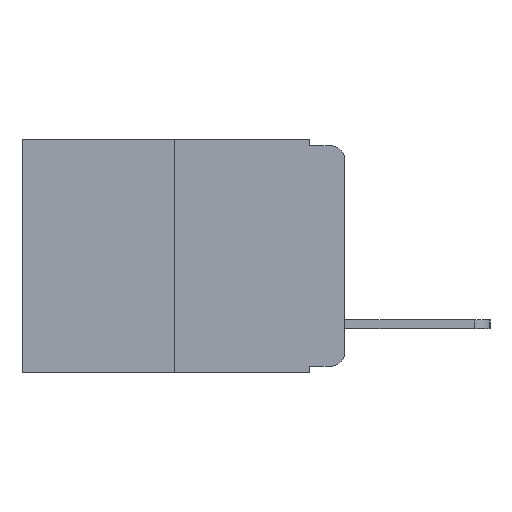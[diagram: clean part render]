
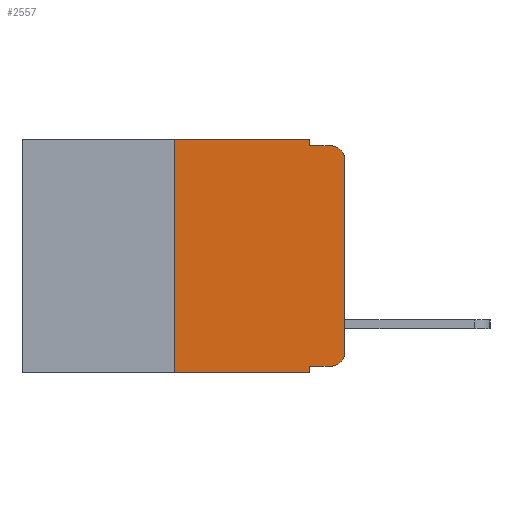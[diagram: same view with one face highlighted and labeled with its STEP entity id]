
A CAD part, left-side view. The second image highlights one B-rep face of the part: STEP entity #2557.
In plain terms, the highlighted planar face has unit normal (-1, 0, 0).
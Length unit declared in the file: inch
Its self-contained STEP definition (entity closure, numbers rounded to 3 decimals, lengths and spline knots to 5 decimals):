
#307 = DIRECTION ( 'NONE',  ( 0., -1., 0. ) ) ;
#320 = EDGE_CURVE ( 'NONE', #17884, #18486, #10785, .T. ) ;
#479 = VERTEX_POINT ( 'NONE', #16959 ) ;
#523 = CARTESIAN_POINT ( 'NONE',  ( 0., 0.051, 0. ) ) ;
#630 = LINE ( 'NONE', #13786, #11543 ) ;
#635 = VECTOR ( 'NONE', #307, 39.37008 ) ;
#1084 = ORIENTED_EDGE ( 'NONE', *, *, #12898, .T. ) ;
#1137 = CARTESIAN_POINT ( 'NONE',  ( 0., 0.473, 0. ) ) ;
#1275 = CIRCLE ( 'NONE', #4536, 0.02 ) ;
#1301 = VERTEX_POINT ( 'NONE', #3215 ) ;
#1553 = DIRECTION ( 'NONE',  ( -1., 0., 0. ) ) ;
#1651 = CARTESIAN_POINT ( 'NONE',  ( 0., 0.051, -0.01 ) ) ;
#2557 = ADVANCED_FACE ( 'NONE', ( #8047 ), #15095, .F. ) ;
#2759 = CARTESIAN_POINT ( 'NONE',  ( 0., 0.051, -0.01 ) ) ;
#2769 = DIRECTION ( 'NONE',  ( 0., 0., 1. ) ) ;
#2838 = VERTEX_POINT ( 'NONE', #18461 ) ;
#2897 = DIRECTION ( 'NONE',  ( 0., -1., 0. ) ) ;
#2990 = DIRECTION ( 'NONE',  ( 0., -1., 0. ) ) ;
#3191 = ORIENTED_EDGE ( 'NONE', *, *, #7468, .F. ) ;
#3215 = CARTESIAN_POINT ( 'NONE',  ( 0., 0.25, 0. ) ) ;
#3253 = ORIENTED_EDGE ( 'NONE', *, *, #10333, .F. ) ;
#3275 = VECTOR ( 'NONE', #9499, 39.37008 ) ;
#3649 = EDGE_CURVE ( 'NONE', #1301, #15613, #4706, .T. ) ;
#4244 = VECTOR ( 'NONE', #2990, 39.37008 ) ;
#4536 = AXIS2_PLACEMENT_3D ( 'NONE', #10446, #1553, #11887 ) ;
#4706 = LINE ( 'NONE', #1137, #4244 ) ;
#5026 = VECTOR ( 'NONE', #17698, 39.37008 ) ;
#5345 = LINE ( 'NONE', #15809, #12645 ) ;
#5619 = CARTESIAN_POINT ( 'NONE',  ( 0., 0.051, 0. ) ) ;
#5855 = CARTESIAN_POINT ( 'NONE',  ( 0., 0.02, -0.03 ) ) ;
#6069 = ORIENTED_EDGE ( 'NONE', *, *, #12273, .T. ) ;
#6139 = CARTESIAN_POINT ( 'NONE',  ( 0., 0.02, -0.333 ) ) ;
#6470 = EDGE_CURVE ( 'NONE', #17884, #9481, #6819, .T. ) ;
#6799 = ORIENTED_EDGE ( 'NONE', *, *, #6470, .F. ) ;
#6819 = LINE ( 'NONE', #523, #3275 ) ;
#7158 = CARTESIAN_POINT ( 'NONE',  ( 0., 0.25, -0.343 ) ) ;
#7377 = DIRECTION ( 'NONE',  ( 0., 0., -1. ) ) ;
#7468 = EDGE_CURVE ( 'NONE', #13738, #1301, #5345, .T. ) ;
#8047 = FACE_OUTER_BOUND ( 'NONE', #12442, .T. ) ;
#8198 = LINE ( 'NONE', #9336, #635 ) ;
#8646 = CARTESIAN_POINT ( 'NONE',  ( 0., 0., -0.313 ) ) ;
#9336 = CARTESIAN_POINT ( 'NONE',  ( 0., 0.473, -0.343 ) ) ;
#9407 = EDGE_CURVE ( 'NONE', #15613, #11278, #12786, .T. ) ;
#9481 = VERTEX_POINT ( 'NONE', #10815 ) ;
#9499 = DIRECTION ( 'NONE',  ( 0., 0., -1. ) ) ;
#9705 = CARTESIAN_POINT ( 'NONE',  ( 0., 0.051, -0.333 ) ) ;
#10333 = EDGE_CURVE ( 'NONE', #11278, #2838, #18729, .T. ) ;
#10446 = CARTESIAN_POINT ( 'NONE',  ( 0., 0.02, -0.313 ) ) ;
#10566 = CARTESIAN_POINT ( 'NONE',  ( 0., 0.051, 0. ) ) ;
#10785 = LINE ( 'NONE', #9705, #18328 ) ;
#10815 = CARTESIAN_POINT ( 'NONE',  ( 0., 0.051, -0.343 ) ) ;
#11278 = VERTEX_POINT ( 'NONE', #2759 ) ;
#11303 = EDGE_CURVE ( 'NONE', #479, #2838, #17561, .T. ) ;
#11543 = VECTOR ( 'NONE', #15211, 39.37008 ) ;
#11887 = DIRECTION ( 'NONE',  ( 0., 0., -1. ) ) ;
#12273 = EDGE_CURVE ( 'NONE', #15795, #479, #630, .T. ) ;
#12442 = EDGE_LOOP ( 'NONE', ( #6069, #18824, #3253, #18166, #14830, #3191, #1084, #6799, #13982, #14456 ) ) ;
#12645 = VECTOR ( 'NONE', #2769, 39.37008 ) ;
#12786 = LINE ( 'NONE', #10566, #5026 ) ;
#12898 = EDGE_CURVE ( 'NONE', #13738, #9481, #8198, .T. ) ;
#13738 = VERTEX_POINT ( 'NONE', #7158 ) ;
#13786 = CARTESIAN_POINT ( 'NONE',  ( 0., 0., 0. ) ) ;
#13936 = CARTESIAN_POINT ( 'NONE',  ( 0., 0.051, -0.333 ) ) ;
#13982 = ORIENTED_EDGE ( 'NONE', *, *, #320, .T. ) ;
#14456 = ORIENTED_EDGE ( 'NONE', *, *, #14549, .T. ) ;
#14549 = EDGE_CURVE ( 'NONE', #18486, #15795, #1275, .T. ) ;
#14567 = VECTOR ( 'NONE', #14915, 39.37008 ) ;
#14830 = ORIENTED_EDGE ( 'NONE', *, *, #3649, .F. ) ;
#14915 = DIRECTION ( 'NONE',  ( 0., -1., 0. ) ) ;
#15095 = PLANE ( 'NONE',  #18398 ) ;
#15209 = DIRECTION ( 'NONE',  ( 0., 0., -1. ) ) ;
#15211 = DIRECTION ( 'NONE',  ( 0., 0., 1. ) ) ;
#15440 = AXIS2_PLACEMENT_3D ( 'NONE', #5855, #15914, #7377 ) ;
#15613 = VERTEX_POINT ( 'NONE', #5619 ) ;
#15795 = VERTEX_POINT ( 'NONE', #8646 ) ;
#15809 = CARTESIAN_POINT ( 'NONE',  ( 0., 0.25, 0. ) ) ;
#15914 = DIRECTION ( 'NONE',  ( -1., 0., 0. ) ) ;
#16959 = CARTESIAN_POINT ( 'NONE',  ( 0., 0., -0.03 ) ) ;
#17561 = CIRCLE ( 'NONE', #15440, 0.02 ) ;
#17698 = DIRECTION ( 'NONE',  ( 0., 0., -1. ) ) ;
#17845 = DIRECTION ( 'NONE',  ( 1., 0., 0. ) ) ;
#17884 = VERTEX_POINT ( 'NONE', #13936 ) ;
#18166 = ORIENTED_EDGE ( 'NONE', *, *, #9407, .F. ) ;
#18328 = VECTOR ( 'NONE', #2897, 39.37008 ) ;
#18398 = AXIS2_PLACEMENT_3D ( 'NONE', #18932, #17845, #15209 ) ;
#18461 = CARTESIAN_POINT ( 'NONE',  ( 0., 0.02, -0.01 ) ) ;
#18486 = VERTEX_POINT ( 'NONE', #6139 ) ;
#18729 = LINE ( 'NONE', #1651, #14567 ) ;
#18824 = ORIENTED_EDGE ( 'NONE', *, *, #11303, .T. ) ;
#18932 = CARTESIAN_POINT ( 'NONE',  ( 0., 0.473, 0. ) ) ;
